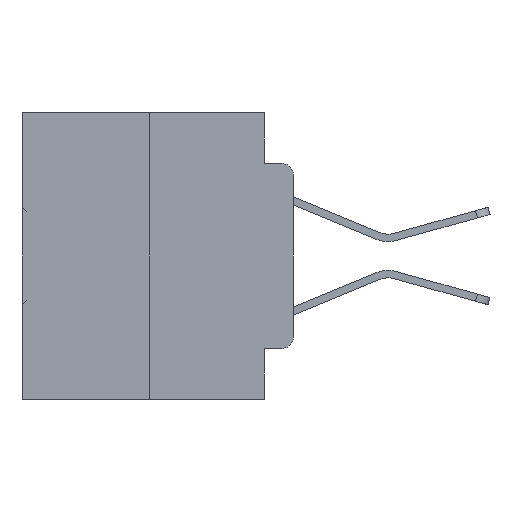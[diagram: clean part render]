
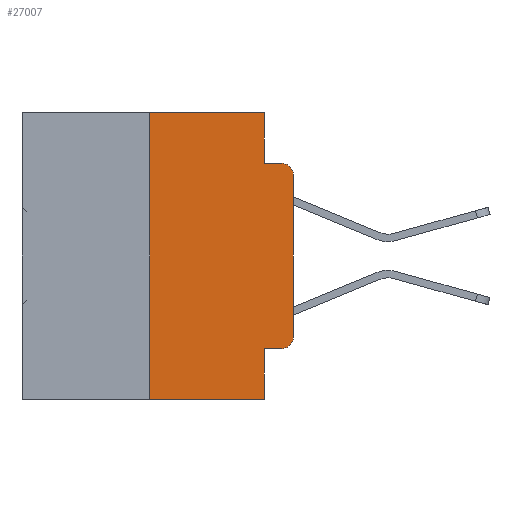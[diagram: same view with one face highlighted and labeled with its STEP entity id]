
A CAD part, left-side view. The second image highlights one B-rep face of the part: STEP entity #27007.
In plain terms, the highlighted planar face has unit normal (-1, 0, 0).
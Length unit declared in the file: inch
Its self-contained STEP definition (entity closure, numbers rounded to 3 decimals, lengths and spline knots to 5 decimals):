
#109 = DIRECTION ( 'NONE',  ( 0., -1., 0. ) ) ;
#439 = EDGE_CURVE ( 'NONE', #17215, #16438, #20769, .T. ) ;
#519 = EDGE_LOOP ( 'NONE', ( #10032, #14233, #18063, #26405, #9078, #31644, #22019, #20513, #31474, #32510 ) ) ;
#1472 = VERTEX_POINT ( 'NONE', #24336 ) ;
#1710 = AXIS2_PLACEMENT_3D ( 'NONE', #29925, #26776, #8504 ) ;
#2092 = CARTESIAN_POINT ( 'NONE',  ( 0., 0.473, 0. ) ) ;
#2125 = LINE ( 'NONE', #34344, #25460 ) ;
#2793 = LINE ( 'NONE', #31715, #17950 ) ;
#2963 = DIRECTION ( 'NONE',  ( -1., 0., 0. ) ) ;
#5077 = CARTESIAN_POINT ( 'NONE',  ( 0., 0.051, -0.4115 ) ) ;
#5150 = EDGE_CURVE ( 'NONE', #16978, #17215, #8156, .T. ) ;
#5185 = EDGE_CURVE ( 'NONE', #18113, #16438, #9993, .T. ) ;
#5294 = DIRECTION ( 'NONE',  ( 0., -1., 0. ) ) ;
#5637 = CARTESIAN_POINT ( 'NONE',  ( 0., 0.051, -0.4115 ) ) ;
#5887 = DIRECTION ( 'NONE',  ( 0., 0., -1. ) ) ;
#6577 = CARTESIAN_POINT ( 'NONE',  ( 0., 0.02, -0.0885 ) ) ;
#7356 = FACE_OUTER_BOUND ( 'NONE', #519, .T. ) ;
#7522 = DIRECTION ( 'NONE',  ( 0., 0., -1. ) ) ;
#8156 = LINE ( 'NONE', #16143, #18384 ) ;
#8190 = LINE ( 'NONE', #11149, #13257 ) ;
#8504 = DIRECTION ( 'NONE',  ( 0., 0., -1. ) ) ;
#8792 = VERTEX_POINT ( 'NONE', #33441 ) ;
#9078 = ORIENTED_EDGE ( 'NONE', *, *, #23046, .F. ) ;
#9993 = CIRCLE ( 'NONE', #1710, 0.02 ) ;
#10032 = ORIENTED_EDGE ( 'NONE', *, *, #25920, .T. ) ;
#10124 = PLANE ( 'NONE',  #15463 ) ;
#10696 = EDGE_CURVE ( 'NONE', #1472, #11697, #32623, .T. ) ;
#11149 = CARTESIAN_POINT ( 'NONE',  ( 0., 0., 0. ) ) ;
#11697 = VERTEX_POINT ( 'NONE', #12462 ) ;
#12367 = VECTOR ( 'NONE', #5294, 39.37008 ) ;
#12462 = CARTESIAN_POINT ( 'NONE',  ( 0., 0.25, 0. ) ) ;
#12751 = DIRECTION ( 'NONE',  ( 0., -1., 0. ) ) ;
#13257 = VECTOR ( 'NONE', #16538, 39.37008 ) ;
#13687 = VERTEX_POINT ( 'NONE', #5077 ) ;
#14172 = DIRECTION ( 'NONE',  ( 0., 0., 1. ) ) ;
#14233 = ORIENTED_EDGE ( 'NONE', *, *, #5185, .T. ) ;
#14579 = CARTESIAN_POINT ( 'NONE',  ( 0., 0.051, -0.0885 ) ) ;
#15463 = AXIS2_PLACEMENT_3D ( 'NONE', #2092, #31535, #7522 ) ;
#15613 = CARTESIAN_POINT ( 'NONE',  ( 0., 0., -0.3915 ) ) ;
#16143 = CARTESIAN_POINT ( 'NONE',  ( 0., 0.051, 0. ) ) ;
#16193 = CARTESIAN_POINT ( 'NONE',  ( 0., 0.02, -0.3915 ) ) ;
#16438 = VERTEX_POINT ( 'NONE', #6577 ) ;
#16538 = DIRECTION ( 'NONE',  ( 0., 0., 1. ) ) ;
#16978 = VERTEX_POINT ( 'NONE', #22194 ) ;
#17137 = AXIS2_PLACEMENT_3D ( 'NONE', #16193, #2963, #26310 ) ;
#17215 = VERTEX_POINT ( 'NONE', #18675 ) ;
#17950 = VECTOR ( 'NONE', #12751, 39.37008 ) ;
#18063 = ORIENTED_EDGE ( 'NONE', *, *, #439, .F. ) ;
#18113 = VERTEX_POINT ( 'NONE', #29706 ) ;
#18384 = VECTOR ( 'NONE', #5887, 39.37008 ) ;
#18570 = LINE ( 'NONE', #34083, #31212 ) ;
#18675 = CARTESIAN_POINT ( 'NONE',  ( 0., 0.051, -0.0885 ) ) ;
#20513 = ORIENTED_EDGE ( 'NONE', *, *, #25337, .F. ) ;
#20633 = EDGE_CURVE ( 'NONE', #33043, #22803, #32153, .T. ) ;
#20769 = LINE ( 'NONE', #14579, #31342 ) ;
#22019 = ORIENTED_EDGE ( 'NONE', *, *, #33318, .T. ) ;
#22194 = CARTESIAN_POINT ( 'NONE',  ( 0., 0.051, 0. ) ) ;
#22803 = VERTEX_POINT ( 'NONE', #15613 ) ;
#23046 = EDGE_CURVE ( 'NONE', #11697, #16978, #18570, .T. ) ;
#24336 = CARTESIAN_POINT ( 'NONE',  ( 0., 0.25, -0.5 ) ) ;
#25337 = EDGE_CURVE ( 'NONE', #13687, #8792, #2125, .T. ) ;
#25460 = VECTOR ( 'NONE', #25988, 39.37008 ) ;
#25920 = EDGE_CURVE ( 'NONE', #22803, #18113, #8190, .T. ) ;
#25987 = DIRECTION ( 'NONE',  ( 0., -1., 0. ) ) ;
#25988 = DIRECTION ( 'NONE',  ( 0., 0., -1. ) ) ;
#26310 = DIRECTION ( 'NONE',  ( 0., 0., -1. ) ) ;
#26405 = ORIENTED_EDGE ( 'NONE', *, *, #5150, .F. ) ;
#26776 = DIRECTION ( 'NONE',  ( -1., 0., 0. ) ) ;
#27007 = ADVANCED_FACE ( 'NONE', ( #7356 ), #10124, .F. ) ;
#29085 = VECTOR ( 'NONE', #14172, 39.37008 ) ;
#29496 = CARTESIAN_POINT ( 'NONE',  ( 0., 0.25, 0. ) ) ;
#29706 = CARTESIAN_POINT ( 'NONE',  ( 0., 0., -0.1085 ) ) ;
#29925 = CARTESIAN_POINT ( 'NONE',  ( 0., 0.02, -0.1085 ) ) ;
#30027 = CARTESIAN_POINT ( 'NONE',  ( 0., 0.02, -0.4115 ) ) ;
#31086 = LINE ( 'NONE', #5637, #12367 ) ;
#31212 = VECTOR ( 'NONE', #109, 39.37008 ) ;
#31342 = VECTOR ( 'NONE', #25987, 39.37008 ) ;
#31474 = ORIENTED_EDGE ( 'NONE', *, *, #32887, .T. ) ;
#31535 = DIRECTION ( 'NONE',  ( 1., 0., 0. ) ) ;
#31644 = ORIENTED_EDGE ( 'NONE', *, *, #10696, .F. ) ;
#31715 = CARTESIAN_POINT ( 'NONE',  ( 0., 0.473, -0.5 ) ) ;
#32153 = CIRCLE ( 'NONE', #17137, 0.02 ) ;
#32510 = ORIENTED_EDGE ( 'NONE', *, *, #20633, .T. ) ;
#32623 = LINE ( 'NONE', #29496, #29085 ) ;
#32887 = EDGE_CURVE ( 'NONE', #13687, #33043, #31086, .T. ) ;
#33043 = VERTEX_POINT ( 'NONE', #30027 ) ;
#33318 = EDGE_CURVE ( 'NONE', #1472, #8792, #2793, .T. ) ;
#33441 = CARTESIAN_POINT ( 'NONE',  ( 0., 0.051, -0.5 ) ) ;
#34083 = CARTESIAN_POINT ( 'NONE',  ( 0., 0.473, 0. ) ) ;
#34344 = CARTESIAN_POINT ( 'NONE',  ( 0., 0.051, 0. ) ) ;
